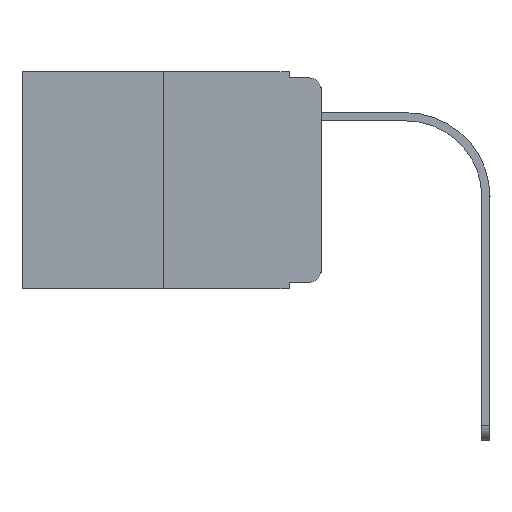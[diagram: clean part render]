
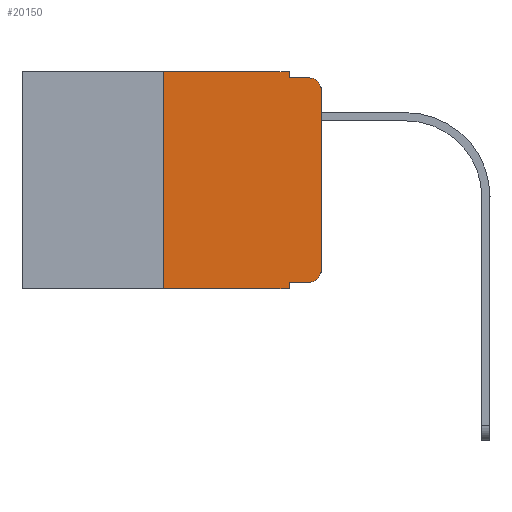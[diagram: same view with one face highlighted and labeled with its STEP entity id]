
A CAD part, left-side view. The second image highlights one B-rep face of the part: STEP entity #20150.
In plain terms, the highlighted planar face has unit normal (-1, 0, 0).
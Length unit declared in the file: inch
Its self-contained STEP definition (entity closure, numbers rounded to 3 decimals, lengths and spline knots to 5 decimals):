
#127 = EDGE_CURVE ( 'NONE', #19715, #14263, #2906, .T. ) ;
#128 = ORIENTED_EDGE ( 'NONE', *, *, #11310, .T. ) ;
#427 = CARTESIAN_POINT ( 'NONE',  ( 0., 0.25, -0.343 ) ) ;
#642 = DIRECTION ( 'NONE',  ( -1., 0., 0. ) ) ;
#939 = DIRECTION ( 'NONE',  ( 0., -1., 0. ) ) ;
#1097 = DIRECTION ( 'NONE',  ( 0., 0., -1. ) ) ;
#1135 = EDGE_CURVE ( 'NONE', #12991, #6363, #20341, .T. ) ;
#1244 = VERTEX_POINT ( 'NONE', #5454 ) ;
#1312 = ORIENTED_EDGE ( 'NONE', *, *, #2872, .T. ) ;
#1675 = VERTEX_POINT ( 'NONE', #1928 ) ;
#1928 = CARTESIAN_POINT ( 'NONE',  ( 0., 0.051, 0. ) ) ;
#2034 = CARTESIAN_POINT ( 'NONE',  ( 0., 0.051, -0.333 ) ) ;
#2201 = AXIS2_PLACEMENT_3D ( 'NONE', #13120, #642, #19416 ) ;
#2233 = ORIENTED_EDGE ( 'NONE', *, *, #127, .T. ) ;
#2563 = VECTOR ( 'NONE', #9496, 39.37008 ) ;
#2624 = LINE ( 'NONE', #9135, #4132 ) ;
#2872 = EDGE_CURVE ( 'NONE', #12991, #11280, #3684, .T. ) ;
#2906 = LINE ( 'NONE', #7446, #3284 ) ;
#3004 = DIRECTION ( 'NONE',  ( 0., 0., -1. ) ) ;
#3075 = VECTOR ( 'NONE', #13044, 39.37008 ) ;
#3284 = VECTOR ( 'NONE', #5680, 39.37008 ) ;
#3439 = LINE ( 'NONE', #17801, #3075 ) ;
#3557 = ORIENTED_EDGE ( 'NONE', *, *, #16142, .F. ) ;
#3684 = LINE ( 'NONE', #2034, #4202 ) ;
#4132 = VECTOR ( 'NONE', #18435, 39.37008 ) ;
#4202 = VECTOR ( 'NONE', #12869, 39.37008 ) ;
#4239 = LINE ( 'NONE', #8884, #7710 ) ;
#4273 = CARTESIAN_POINT ( 'NONE',  ( 0., 0.25, 0. ) ) ;
#4299 = CARTESIAN_POINT ( 'NONE',  ( 0., 0.473, 0. ) ) ;
#4790 = CIRCLE ( 'NONE', #10079, 0.02 ) ;
#4794 = EDGE_CURVE ( 'NONE', #19465, #6363, #4239, .T. ) ;
#5204 = DIRECTION ( 'NONE',  ( -1., 0., 0. ) ) ;
#5358 = CARTESIAN_POINT ( 'NONE',  ( 0., 0.02, -0.333 ) ) ;
#5454 = CARTESIAN_POINT ( 'NONE',  ( 0., 0.051, -0.01 ) ) ;
#5680 = DIRECTION ( 'NONE',  ( 0., 0., 1. ) ) ;
#5941 = PLANE ( 'NONE',  #19305 ) ;
#6188 = CARTESIAN_POINT ( 'NONE',  ( 0., 0.051, 0. ) ) ;
#6189 = ORIENTED_EDGE ( 'NONE', *, *, #7207, .F. ) ;
#6363 = VERTEX_POINT ( 'NONE', #19502 ) ;
#6383 = ORIENTED_EDGE ( 'NONE', *, *, #4794, .T. ) ;
#7207 = EDGE_CURVE ( 'NONE', #1244, #18119, #3439, .T. ) ;
#7446 = CARTESIAN_POINT ( 'NONE',  ( 0., 0., 0. ) ) ;
#7707 = CARTESIAN_POINT ( 'NONE',  ( 0., 0., -0.313 ) ) ;
#7710 = VECTOR ( 'NONE', #939, 39.37008 ) ;
#7715 = VECTOR ( 'NONE', #3004, 39.37008 ) ;
#8884 = CARTESIAN_POINT ( 'NONE',  ( 0., 0.473, -0.343 ) ) ;
#9135 = CARTESIAN_POINT ( 'NONE',  ( 0., 0.25, 0. ) ) ;
#9391 = CARTESIAN_POINT ( 'NONE',  ( 0., 0.02, -0.01 ) ) ;
#9462 = ORIENTED_EDGE ( 'NONE', *, *, #10647, .F. ) ;
#9496 = DIRECTION ( 'NONE',  ( 0., 0., -1. ) ) ;
#9681 = ORIENTED_EDGE ( 'NONE', *, *, #17176, .T. ) ;
#9765 = LINE ( 'NONE', #17422, #17550 ) ;
#10079 = AXIS2_PLACEMENT_3D ( 'NONE', #14729, #5204, #16172 ) ;
#10236 = CARTESIAN_POINT ( 'NONE',  ( 0., 0.051, -0.333 ) ) ;
#10647 = EDGE_CURVE ( 'NONE', #19465, #17543, #2624, .T. ) ;
#11280 = VERTEX_POINT ( 'NONE', #5358 ) ;
#11310 = EDGE_CURVE ( 'NONE', #11280, #19715, #12402, .T. ) ;
#12402 = CIRCLE ( 'NONE', #2201, 0.02 ) ;
#12548 = DIRECTION ( 'NONE',  ( 0., -1., 0. ) ) ;
#12704 = LINE ( 'NONE', #19018, #7715 ) ;
#12869 = DIRECTION ( 'NONE',  ( 0., -1., 0. ) ) ;
#12991 = VERTEX_POINT ( 'NONE', #10236 ) ;
#13044 = DIRECTION ( 'NONE',  ( 0., -1., 0. ) ) ;
#13120 = CARTESIAN_POINT ( 'NONE',  ( 0., 0.02, -0.313 ) ) ;
#13987 = EDGE_CURVE ( 'NONE', #17543, #1675, #9765, .T. ) ;
#14245 = ORIENTED_EDGE ( 'NONE', *, *, #1135, .F. ) ;
#14263 = VERTEX_POINT ( 'NONE', #15146 ) ;
#14729 = CARTESIAN_POINT ( 'NONE',  ( 0., 0.02, -0.03 ) ) ;
#15146 = CARTESIAN_POINT ( 'NONE',  ( 0., 0., -0.03 ) ) ;
#16142 = EDGE_CURVE ( 'NONE', #1675, #1244, #12704, .T. ) ;
#16172 = DIRECTION ( 'NONE',  ( 0., 0., -1. ) ) ;
#17176 = EDGE_CURVE ( 'NONE', #14263, #18119, #4790, .T. ) ;
#17422 = CARTESIAN_POINT ( 'NONE',  ( 0., 0.473, 0. ) ) ;
#17543 = VERTEX_POINT ( 'NONE', #4273 ) ;
#17550 = VECTOR ( 'NONE', #12548, 39.37008 ) ;
#17801 = CARTESIAN_POINT ( 'NONE',  ( 0., 0.051, -0.01 ) ) ;
#17825 = ORIENTED_EDGE ( 'NONE', *, *, #13987, .F. ) ;
#18119 = VERTEX_POINT ( 'NONE', #9391 ) ;
#18221 = EDGE_LOOP ( 'NONE', ( #2233, #9681, #6189, #3557, #17825, #9462, #6383, #14245, #1312, #128 ) ) ;
#18435 = DIRECTION ( 'NONE',  ( 0., 0., 1. ) ) ;
#18554 = FACE_OUTER_BOUND ( 'NONE', #18221, .T. ) ;
#19018 = CARTESIAN_POINT ( 'NONE',  ( 0., 0.051, 0. ) ) ;
#19305 = AXIS2_PLACEMENT_3D ( 'NONE', #4299, #20296, #1097 ) ;
#19416 = DIRECTION ( 'NONE',  ( 0., 0., -1. ) ) ;
#19465 = VERTEX_POINT ( 'NONE', #427 ) ;
#19502 = CARTESIAN_POINT ( 'NONE',  ( 0., 0.051, -0.343 ) ) ;
#19715 = VERTEX_POINT ( 'NONE', #7707 ) ;
#20150 = ADVANCED_FACE ( 'NONE', ( #18554 ), #5941, .F. ) ;
#20296 = DIRECTION ( 'NONE',  ( 1., 0., 0. ) ) ;
#20341 = LINE ( 'NONE', #6188, #2563 ) ;
